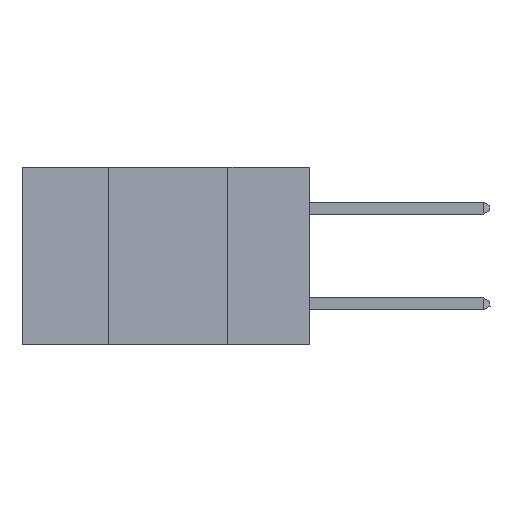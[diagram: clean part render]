
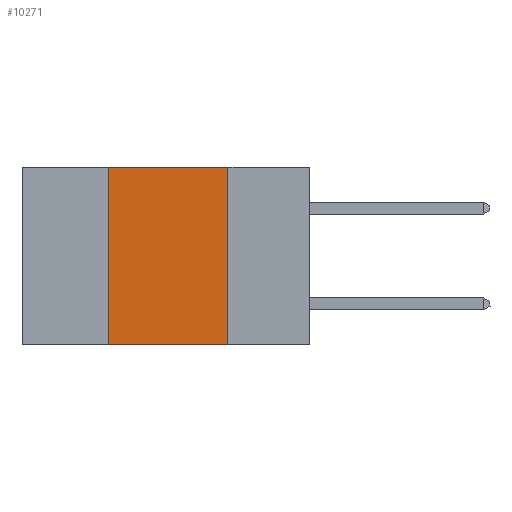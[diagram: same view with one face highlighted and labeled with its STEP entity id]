
A CAD part, left-side view. The second image highlights one B-rep face of the part: STEP entity #10271.
In plain terms, the highlighted planar face has unit normal (-1, 0, 0).
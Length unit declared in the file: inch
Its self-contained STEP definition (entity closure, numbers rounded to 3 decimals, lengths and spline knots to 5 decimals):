
#289 = PLANE ( 'NONE',  #5230 ) ;
#4194 = DIRECTION ( 'NONE',  ( 1., 0., 0. ) ) ;
#4258 = DIRECTION ( 'NONE',  ( 0., -1., 0. ) ) ;
#4450 = EDGE_CURVE ( 'NONE', #20802, #16251, #4989, .T. ) ;
#4989 = LINE ( 'NONE', #17201, #17754 ) ;
#5046 = VERTEX_POINT ( 'NONE', #18849 ) ;
#5230 = AXIS2_PLACEMENT_3D ( 'NONE', #15631, #4194, #19108 ) ;
#5744 = VECTOR ( 'NONE', #4258, 39.37008 ) ;
#5762 = DIRECTION ( 'NONE',  ( 0., -1., 0. ) ) ;
#8915 = EDGE_CURVE ( 'NONE', #5046, #16251, #19061, .T. ) ;
#9419 = EDGE_CURVE ( 'NONE', #20802, #10289, #19038, .T. ) ;
#10271 = ADVANCED_FACE ( 'NONE', ( #11296 ), #289, .F. ) ;
#10289 = VERTEX_POINT ( 'NONE', #19346 ) ;
#10318 = DIRECTION ( 'NONE',  ( 0., 0., 1. ) ) ;
#11296 = FACE_OUTER_BOUND ( 'NONE', #21858, .T. ) ;
#12162 = CARTESIAN_POINT ( 'NONE',  ( 0., 0.42, -0.37 ) ) ;
#14000 = VECTOR ( 'NONE', #10318, 39.37008 ) ;
#14015 = ORIENTED_EDGE ( 'NONE', *, *, #4450, .T. ) ;
#15615 = ORIENTED_EDGE ( 'NONE', *, *, #9419, .F. ) ;
#15631 = CARTESIAN_POINT ( 'NONE',  ( 0., 0.6, 0. ) ) ;
#15984 = CARTESIAN_POINT ( 'NONE',  ( 0., 0.17, -0.37 ) ) ;
#16251 = VERTEX_POINT ( 'NONE', #15984 ) ;
#16541 = DIRECTION ( 'NONE',  ( 0., 0., -1. ) ) ;
#17129 = EDGE_CURVE ( 'NONE', #10289, #5046, #24462, .T. ) ;
#17201 = CARTESIAN_POINT ( 'NONE',  ( 0., 0.6, -0.37 ) ) ;
#17754 = VECTOR ( 'NONE', #5762, 39.37008 ) ;
#17802 = CARTESIAN_POINT ( 'NONE',  ( 0., 0.6, 0. ) ) ;
#18441 = CARTESIAN_POINT ( 'NONE',  ( 0., 0.17, 0. ) ) ;
#18849 = CARTESIAN_POINT ( 'NONE',  ( 0., 0.17, 0. ) ) ;
#19038 = LINE ( 'NONE', #21695, #14000 ) ;
#19061 = LINE ( 'NONE', #18441, #21468 ) ;
#19108 = DIRECTION ( 'NONE',  ( 0., 0., -1. ) ) ;
#19280 = ORIENTED_EDGE ( 'NONE', *, *, #8915, .F. ) ;
#19346 = CARTESIAN_POINT ( 'NONE',  ( 0., 0.42, 0. ) ) ;
#19863 = ORIENTED_EDGE ( 'NONE', *, *, #17129, .F. ) ;
#20802 = VERTEX_POINT ( 'NONE', #12162 ) ;
#21468 = VECTOR ( 'NONE', #16541, 39.37008 ) ;
#21695 = CARTESIAN_POINT ( 'NONE',  ( 0., 0.42, 0. ) ) ;
#21858 = EDGE_LOOP ( 'NONE', ( #19280, #19863, #15615, #14015 ) ) ;
#24462 = LINE ( 'NONE', #17802, #5744 ) ;
